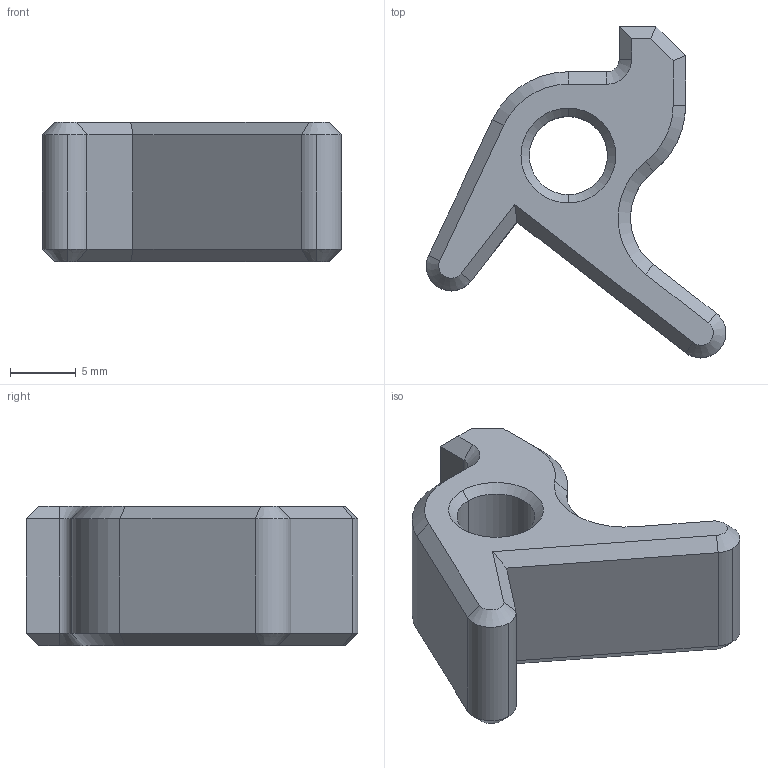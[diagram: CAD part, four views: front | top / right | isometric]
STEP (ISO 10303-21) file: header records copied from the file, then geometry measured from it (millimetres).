
FILE_DESCRIPTION (( 'STEP AP203' ), '1' );
FILE_NAME ('AF-HF-AS-PRT-001-STEP.STEP', '2020-10-04T16:21:39', ( '' ), ( '' ), 'SwSTEP 2.0', 'SolidWorks 2018', '' );
FILE_SCHEMA (( 'CONFIG_CONTROL_DESIGN' ));
Length unit declared in the file: inch
Products named in the file (1): AF-HF-AS-PRT-001-STEP
Bounding box: 22.84 x 25.32 x 10.63 mm (x, y, z)
Volume: 2361.7 mm3; surface area: 1491.3 mm2
Topology: 1 solids, 1 shells, 60 faces, 137 edges, 79 vertices
Faces by surface type: plane 29, cone 20, cylinder 11
Entity records: 1731 total; most frequent: DIRECTION 302, CARTESIAN_POINT 277, ORIENTED_EDGE 274, EDGE_CURVE 137, AXIS2_PLACEMENT_3D 104, VECTOR 94, LINE 94, VERTEX_POINT 79
